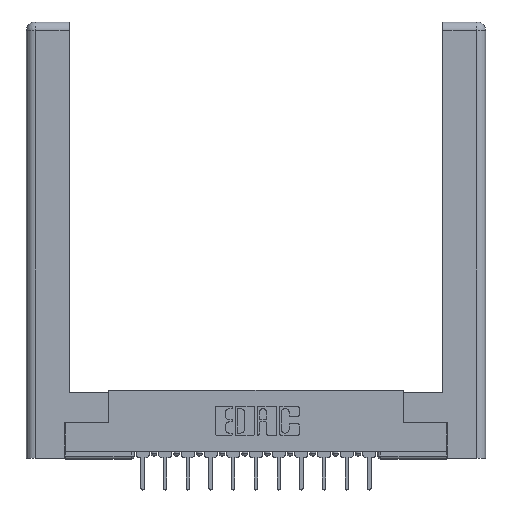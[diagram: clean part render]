
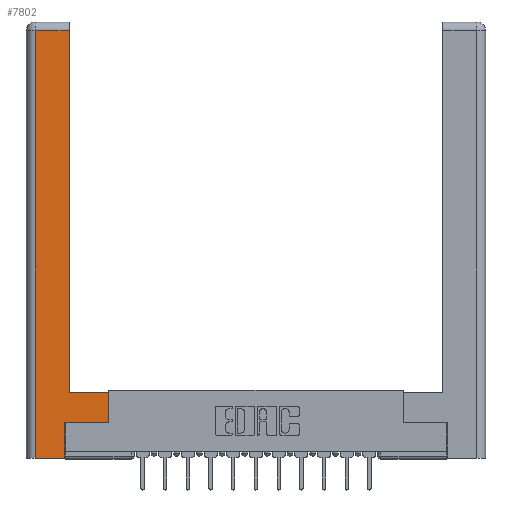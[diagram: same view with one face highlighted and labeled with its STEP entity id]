
A CAD part, top view. The second image highlights one B-rep face of the part: STEP entity #7802.
In plain terms, the highlighted planar face has unit normal (0, 0, 1).
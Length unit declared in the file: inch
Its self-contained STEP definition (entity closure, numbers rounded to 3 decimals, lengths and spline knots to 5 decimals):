
#49 = PLANE ( 'NONE',  #4546 ) ;
#275 = VECTOR ( 'NONE', #10469, 39.37008 ) ;
#444 = CARTESIAN_POINT ( 'NONE',  ( 0.295, 0.45, 0. ) ) ;
#801 = VERTEX_POINT ( 'NONE', #444 ) ;
#828 = DIRECTION ( 'NONE',  ( 1., 0., 0. ) ) ;
#834 = DIRECTION ( 'NONE',  ( -1., 0., 0. ) ) ;
#1113 = LINE ( 'NONE', #9712, #10040 ) ;
#1215 = DIRECTION ( 'NONE',  ( 0., -1., 0. ) ) ;
#1431 = VERTEX_POINT ( 'NONE', #15007 ) ;
#1925 = EDGE_CURVE ( 'NONE', #1431, #4290, #3586, .T. ) ;
#1976 = EDGE_CURVE ( 'NONE', #7582, #1431, #14152, .T. ) ;
#2217 = ORIENTED_EDGE ( 'NONE', *, *, #1925, .T. ) ;
#2718 = VERTEX_POINT ( 'NONE', #6187 ) ;
#2922 = ORIENTED_EDGE ( 'NONE', *, *, #9986, .T. ) ;
#3043 = CARTESIAN_POINT ( 'NONE',  ( 0.0615, 0., 0. ) ) ;
#3408 = CARTESIAN_POINT ( 'NONE',  ( 0.265, 0.245, 0. ) ) ;
#3586 = LINE ( 'NONE', #13606, #11045 ) ;
#3593 = VECTOR ( 'NONE', #14864, 39.37008 ) ;
#4267 = EDGE_CURVE ( 'NONE', #4290, #11802, #9204, .T. ) ;
#4290 = VERTEX_POINT ( 'NONE', #3043 ) ;
#4520 = LINE ( 'NONE', #15523, #5663 ) ;
#4546 = AXIS2_PLACEMENT_3D ( 'NONE', #8757, #12468, #15073 ) ;
#4715 = ORIENTED_EDGE ( 'NONE', *, *, #12760, .T. ) ;
#5033 = EDGE_CURVE ( 'NONE', #801, #7582, #1113, .T. ) ;
#5663 = VECTOR ( 'NONE', #834, 39.37008 ) ;
#5819 = ORIENTED_EDGE ( 'NONE', *, *, #1976, .T. ) ;
#6003 = VECTOR ( 'NONE', #15885, 39.37008 ) ;
#6147 = EDGE_CURVE ( 'NONE', #11802, #6269, #8000, .T. ) ;
#6184 = CARTESIAN_POINT ( 'NONE',  ( 0.565, 0.45, 0. ) ) ;
#6187 = CARTESIAN_POINT ( 'NONE',  ( 0.565, 0.45, 0. ) ) ;
#6269 = VERTEX_POINT ( 'NONE', #3408 ) ;
#6547 = EDGE_LOOP ( 'NONE', ( #16081, #5819, #2217, #13773, #8898, #10216, #4715, #2922 ) ) ;
#6896 = LINE ( 'NONE', #9590, #9143 ) ;
#7582 = VERTEX_POINT ( 'NONE', #7940 ) ;
#7782 = VERTEX_POINT ( 'NONE', #12627 ) ;
#7802 = ADVANCED_FACE ( 'NONE', ( #10454 ), #49, .F. ) ;
#7940 = CARTESIAN_POINT ( 'NONE',  ( 0.295, 2.94, 0. ) ) ;
#8000 = LINE ( 'NONE', #13014, #6003 ) ;
#8757 = CARTESIAN_POINT ( 'NONE',  ( 0., 0., 0. ) ) ;
#8898 = ORIENTED_EDGE ( 'NONE', *, *, #6147, .T. ) ;
#9143 = VECTOR ( 'NONE', #15926, 39.37008 ) ;
#9204 = LINE ( 'NONE', #14195, #13050 ) ;
#9431 = CARTESIAN_POINT ( 'NONE',  ( 0.265, 0., 0. ) ) ;
#9590 = CARTESIAN_POINT ( 'NONE',  ( 0.565, 0.245, 0. ) ) ;
#9692 = LINE ( 'NONE', #6184, #3593 ) ;
#9712 = CARTESIAN_POINT ( 'NONE',  ( 0.295, 3., 0. ) ) ;
#9986 = EDGE_CURVE ( 'NONE', #2718, #801, #4520, .T. ) ;
#10040 = VECTOR ( 'NONE', #12437, 39.37008 ) ;
#10216 = ORIENTED_EDGE ( 'NONE', *, *, #14409, .T. ) ;
#10454 = FACE_OUTER_BOUND ( 'NONE', #6547, .T. ) ;
#10469 = DIRECTION ( 'NONE',  ( -1., 0., 0. ) ) ;
#11045 = VECTOR ( 'NONE', #1215, 39.37008 ) ;
#11802 = VERTEX_POINT ( 'NONE', #9431 ) ;
#12437 = DIRECTION ( 'NONE',  ( 0., 1., 0. ) ) ;
#12468 = DIRECTION ( 'NONE',  ( 0., 0., -1. ) ) ;
#12627 = CARTESIAN_POINT ( 'NONE',  ( 0.565, 0.245, 0. ) ) ;
#12760 = EDGE_CURVE ( 'NONE', #7782, #2718, #9692, .T. ) ;
#13014 = CARTESIAN_POINT ( 'NONE',  ( 0.265, 0.245, 0. ) ) ;
#13050 = VECTOR ( 'NONE', #828, 39.37008 ) ;
#13606 = CARTESIAN_POINT ( 'NONE',  ( 0.0615, 0., 0. ) ) ;
#13773 = ORIENTED_EDGE ( 'NONE', *, *, #4267, .T. ) ;
#13996 = CARTESIAN_POINT ( 'NONE',  ( 0.0615, 2.94, 0. ) ) ;
#14152 = LINE ( 'NONE', #13996, #275 ) ;
#14195 = CARTESIAN_POINT ( 'NONE',  ( 0.265, 0., 0. ) ) ;
#14409 = EDGE_CURVE ( 'NONE', #6269, #7782, #6896, .T. ) ;
#14864 = DIRECTION ( 'NONE',  ( 0., 1., 0. ) ) ;
#15007 = CARTESIAN_POINT ( 'NONE',  ( 0.0615, 2.94, 0. ) ) ;
#15073 = DIRECTION ( 'NONE',  ( -1., 0., 0. ) ) ;
#15523 = CARTESIAN_POINT ( 'NONE',  ( 0.295, 0.45, 0. ) ) ;
#15885 = DIRECTION ( 'NONE',  ( 0., 1., 0. ) ) ;
#15926 = DIRECTION ( 'NONE',  ( 1., 0., 0. ) ) ;
#16081 = ORIENTED_EDGE ( 'NONE', *, *, #5033, .T. ) ;
